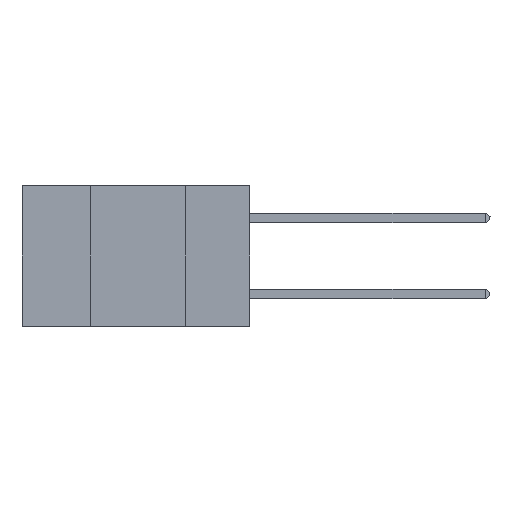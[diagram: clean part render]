
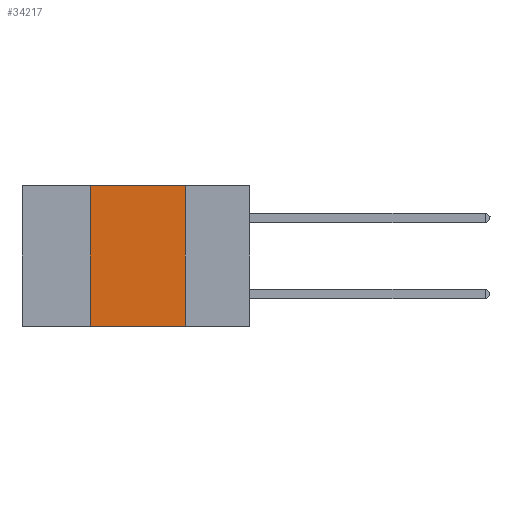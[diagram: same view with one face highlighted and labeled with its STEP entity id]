
A CAD part, left-side view. The second image highlights one B-rep face of the part: STEP entity #34217.
In plain terms, the highlighted planar face has unit normal (-1, 0, 0).
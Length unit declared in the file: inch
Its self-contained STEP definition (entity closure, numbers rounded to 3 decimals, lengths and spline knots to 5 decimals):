
#290 = DIRECTION ( 'NONE',  ( 0., -1., 0. ) ) ;
#1950 = CARTESIAN_POINT ( 'NONE',  ( 0., 0.6, -0.37 ) ) ;
#3586 = CARTESIAN_POINT ( 'NONE',  ( 0., 0.6, 0. ) ) ;
#3811 = CARTESIAN_POINT ( 'NONE',  ( 0., 0.42, -0.37 ) ) ;
#6046 = VECTOR ( 'NONE', #35263, 39.37008 ) ;
#6620 = LINE ( 'NONE', #13000, #6046 ) ;
#6708 = DIRECTION ( 'NONE',  ( 0., 0., 1. ) ) ;
#7945 = VERTEX_POINT ( 'NONE', #13576 ) ;
#9921 = FACE_OUTER_BOUND ( 'NONE', #21424, .T. ) ;
#10563 = VECTOR ( 'NONE', #6708, 39.37008 ) ;
#10671 = ORIENTED_EDGE ( 'NONE', *, *, #34190, .F. ) ;
#11331 = EDGE_CURVE ( 'NONE', #29466, #7945, #29780, .T. ) ;
#13000 = CARTESIAN_POINT ( 'NONE',  ( 0., 0.17, 0. ) ) ;
#13576 = CARTESIAN_POINT ( 'NONE',  ( 0., 0.17, -0.37 ) ) ;
#15633 = VERTEX_POINT ( 'NONE', #38349 ) ;
#19072 = CARTESIAN_POINT ( 'NONE',  ( 0., 0.42, 0. ) ) ;
#19730 = VERTEX_POINT ( 'NONE', #37968 ) ;
#19787 = CARTESIAN_POINT ( 'NONE',  ( 0., 0.6, 0. ) ) ;
#20155 = VECTOR ( 'NONE', #290, 39.37008 ) ;
#21424 = EDGE_LOOP ( 'NONE', ( #10671, #33520, #22374, #35197 ) ) ;
#22374 = ORIENTED_EDGE ( 'NONE', *, *, #32446, .F. ) ;
#22642 = EDGE_CURVE ( 'NONE', #15633, #19730, #32442, .T. ) ;
#26189 = PLANE ( 'NONE',  #37622 ) ;
#29466 = VERTEX_POINT ( 'NONE', #3811 ) ;
#29780 = LINE ( 'NONE', #1950, #38214 ) ;
#32162 = DIRECTION ( 'NONE',  ( 0., 0., -1. ) ) ;
#32442 = LINE ( 'NONE', #3586, #20155 ) ;
#32446 = EDGE_CURVE ( 'NONE', #29466, #15633, #38002, .T. ) ;
#33520 = ORIENTED_EDGE ( 'NONE', *, *, #22642, .F. ) ;
#34190 = EDGE_CURVE ( 'NONE', #19730, #7945, #6620, .T. ) ;
#34217 = ADVANCED_FACE ( 'NONE', ( #9921 ), #26189, .F. ) ;
#35197 = ORIENTED_EDGE ( 'NONE', *, *, #11331, .T. ) ;
#35263 = DIRECTION ( 'NONE',  ( 0., 0., -1. ) ) ;
#36166 = DIRECTION ( 'NONE',  ( 0., -1., 0. ) ) ;
#37622 = AXIS2_PLACEMENT_3D ( 'NONE', #19787, #37925, #32162 ) ;
#37925 = DIRECTION ( 'NONE',  ( 1., 0., 0. ) ) ;
#37968 = CARTESIAN_POINT ( 'NONE',  ( 0., 0.17, 0. ) ) ;
#38002 = LINE ( 'NONE', #19072, #10563 ) ;
#38214 = VECTOR ( 'NONE', #36166, 39.37008 ) ;
#38349 = CARTESIAN_POINT ( 'NONE',  ( 0., 0.42, 0. ) ) ;
